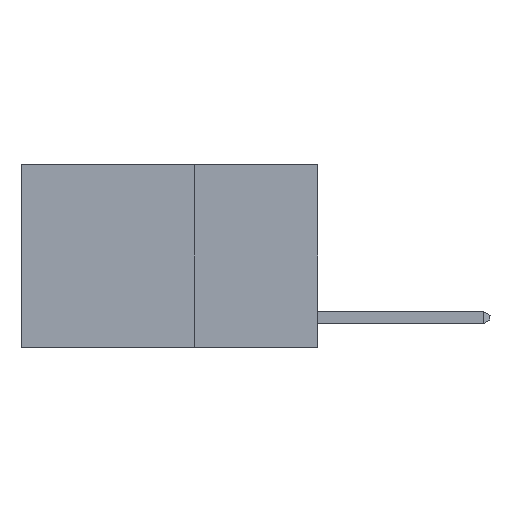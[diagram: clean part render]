
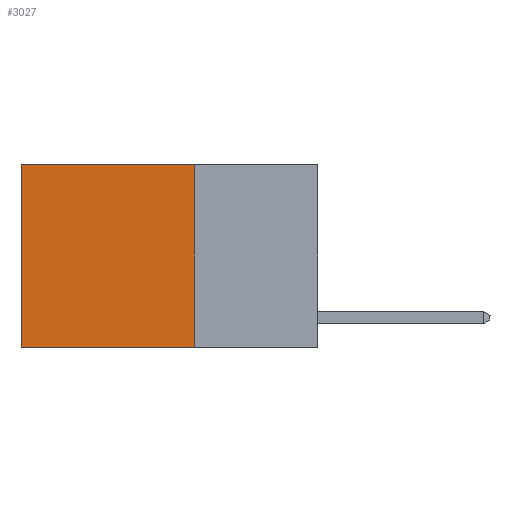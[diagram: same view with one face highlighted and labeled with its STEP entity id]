
A CAD part, left-side view. The second image highlights one B-rep face of the part: STEP entity #3027.
In plain terms, the highlighted planar face has unit normal (-1, 0, 0).
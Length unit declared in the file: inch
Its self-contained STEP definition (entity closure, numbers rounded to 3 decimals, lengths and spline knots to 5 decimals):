
#401 = CARTESIAN_POINT ( 'NONE',  ( 0.2625, 0.25, 0. ) ) ;
#1223 = DIRECTION ( 'NONE',  ( 0., 1., 0. ) ) ;
#2402 = ORIENTED_EDGE ( 'NONE', *, *, #11301, .T. ) ;
#2426 = EDGE_CURVE ( 'NONE', #3644, #10921, #9028, .T. ) ;
#2709 = VECTOR ( 'NONE', #5576, 39.37008 ) ;
#2728 = CARTESIAN_POINT ( 'NONE',  ( 0.2625, 0.25, 0. ) ) ;
#3027 = ADVANCED_FACE ( 'NONE', ( #9120 ), #3900, .F. ) ;
#3089 = LINE ( 'NONE', #13443, #6873 ) ;
#3602 = LINE ( 'NONE', #2728, #3768 ) ;
#3644 = VERTEX_POINT ( 'NONE', #401 ) ;
#3768 = VECTOR ( 'NONE', #8134, 39.37008 ) ;
#3900 = PLANE ( 'NONE',  #7752 ) ;
#4690 = CARTESIAN_POINT ( 'NONE',  ( 0.2625, 0.25, -0.37 ) ) ;
#5074 = ORIENTED_EDGE ( 'NONE', *, *, #5243, .F. ) ;
#5150 = EDGE_CURVE ( 'NONE', #3644, #14394, #3602, .T. ) ;
#5243 = EDGE_CURVE ( 'NONE', #10921, #5756, #3089, .T. ) ;
#5576 = DIRECTION ( 'NONE',  ( 0., 0., -1. ) ) ;
#5756 = VERTEX_POINT ( 'NONE', #8863 ) ;
#6299 = LINE ( 'NONE', #12312, #2709 ) ;
#6873 = VECTOR ( 'NONE', #1223, 39.37008 ) ;
#7039 = VECTOR ( 'NONE', #9291, 39.37008 ) ;
#7235 = CARTESIAN_POINT ( 'NONE',  ( 0.2625, 0.25, 0. ) ) ;
#7621 = ORIENTED_EDGE ( 'NONE', *, *, #5150, .T. ) ;
#7752 = AXIS2_PLACEMENT_3D ( 'NONE', #7235, #10694, #10584 ) ;
#8125 = CARTESIAN_POINT ( 'NONE',  ( 0.2625, 0.25, 0. ) ) ;
#8134 = DIRECTION ( 'NONE',  ( 0., 1., 0. ) ) ;
#8358 = EDGE_LOOP ( 'NONE', ( #2402, #5074, #13057, #7621 ) ) ;
#8863 = CARTESIAN_POINT ( 'NONE',  ( 0.2625, 0.6, -0.37 ) ) ;
#9028 = LINE ( 'NONE', #8125, #7039 ) ;
#9120 = FACE_OUTER_BOUND ( 'NONE', #8358, .T. ) ;
#9291 = DIRECTION ( 'NONE',  ( 0., 0., -1. ) ) ;
#10584 = DIRECTION ( 'NONE',  ( 0., 0., -1. ) ) ;
#10694 = DIRECTION ( 'NONE',  ( 1., 0., 0. ) ) ;
#10921 = VERTEX_POINT ( 'NONE', #4690 ) ;
#11301 = EDGE_CURVE ( 'NONE', #14394, #5756, #6299, .T. ) ;
#12312 = CARTESIAN_POINT ( 'NONE',  ( 0.2625, 0.6, 0. ) ) ;
#13057 = ORIENTED_EDGE ( 'NONE', *, *, #2426, .F. ) ;
#13443 = CARTESIAN_POINT ( 'NONE',  ( 0.2625, 0.25, -0.37 ) ) ;
#13654 = CARTESIAN_POINT ( 'NONE',  ( 0.2625, 0.6, 0. ) ) ;
#14394 = VERTEX_POINT ( 'NONE', #13654 ) ;
